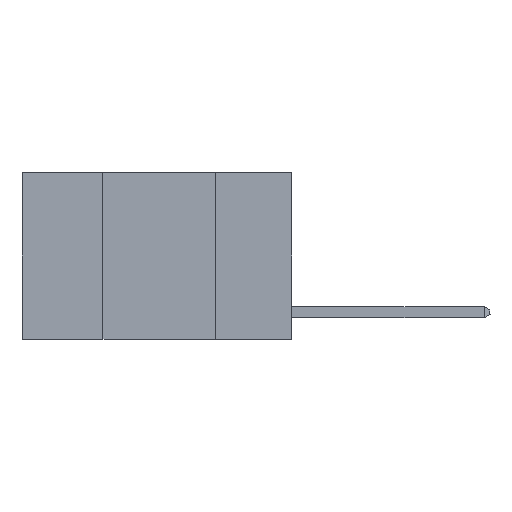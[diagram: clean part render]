
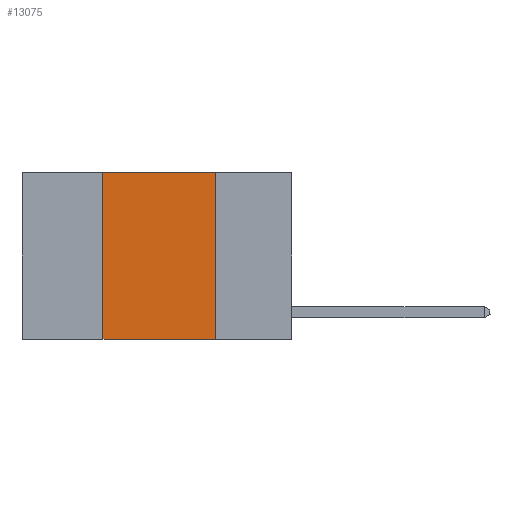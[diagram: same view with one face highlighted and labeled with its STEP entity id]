
A CAD part, left-side view. The second image highlights one B-rep face of the part: STEP entity #13075.
In plain terms, the highlighted planar face has unit normal (-1, 0, 0).
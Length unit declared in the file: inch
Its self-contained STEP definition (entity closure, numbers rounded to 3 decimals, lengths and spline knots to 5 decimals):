
#274 = VECTOR ( 'NONE', #16319, 39.37008 ) ;
#1256 = LINE ( 'NONE', #19214, #22501 ) ;
#1364 = CARTESIAN_POINT ( 'NONE',  ( 0., 0.17, 0. ) ) ;
#1908 = LINE ( 'NONE', #15973, #274 ) ;
#2144 = DIRECTION ( 'NONE',  ( 0., -1., 0. ) ) ;
#2211 = CARTESIAN_POINT ( 'NONE',  ( 0., 0.6, 0. ) ) ;
#2623 = CARTESIAN_POINT ( 'NONE',  ( 0., 0.42, 0. ) ) ;
#2859 = ORIENTED_EDGE ( 'NONE', *, *, #5533, .F. ) ;
#3332 = PLANE ( 'NONE',  #6863 ) ;
#3520 = ORIENTED_EDGE ( 'NONE', *, *, #22010, .F. ) ;
#4323 = VERTEX_POINT ( 'NONE', #11855 ) ;
#4763 = VERTEX_POINT ( 'NONE', #1364 ) ;
#4826 = CARTESIAN_POINT ( 'NONE',  ( 0., 0.6, 0. ) ) ;
#5484 = VECTOR ( 'NONE', #10722, 39.37008 ) ;
#5533 = EDGE_CURVE ( 'NONE', #20583, #4763, #5913, .T. ) ;
#5913 = LINE ( 'NONE', #2211, #5484 ) ;
#6428 = EDGE_CURVE ( 'NONE', #4323, #20583, #1256, .T. ) ;
#6863 = AXIS2_PLACEMENT_3D ( 'NONE', #4826, #11862, #8511 ) ;
#8511 = DIRECTION ( 'NONE',  ( 0., 0., -1. ) ) ;
#9166 = ORIENTED_EDGE ( 'NONE', *, *, #12781, .T. ) ;
#9820 = VECTOR ( 'NONE', #2144, 39.37008 ) ;
#10216 = ORIENTED_EDGE ( 'NONE', *, *, #6428, .F. ) ;
#10437 = DIRECTION ( 'NONE',  ( 0., 0., 1. ) ) ;
#10722 = DIRECTION ( 'NONE',  ( 0., -1., 0. ) ) ;
#11855 = CARTESIAN_POINT ( 'NONE',  ( 0., 0.42, -0.37 ) ) ;
#11862 = DIRECTION ( 'NONE',  ( 1., 0., 0. ) ) ;
#12766 = CARTESIAN_POINT ( 'NONE',  ( 0., 0.6, -0.37 ) ) ;
#12781 = EDGE_CURVE ( 'NONE', #4323, #16736, #14486, .T. ) ;
#13075 = ADVANCED_FACE ( 'NONE', ( #20639 ), #3332, .F. ) ;
#13975 = CARTESIAN_POINT ( 'NONE',  ( 0., 0.17, -0.37 ) ) ;
#14486 = LINE ( 'NONE', #12766, #9820 ) ;
#15973 = CARTESIAN_POINT ( 'NONE',  ( 0., 0.17, 0. ) ) ;
#16319 = DIRECTION ( 'NONE',  ( 0., 0., -1. ) ) ;
#16736 = VERTEX_POINT ( 'NONE', #13975 ) ;
#18454 = EDGE_LOOP ( 'NONE', ( #3520, #2859, #10216, #9166 ) ) ;
#19214 = CARTESIAN_POINT ( 'NONE',  ( 0., 0.42, 0. ) ) ;
#20583 = VERTEX_POINT ( 'NONE', #2623 ) ;
#20639 = FACE_OUTER_BOUND ( 'NONE', #18454, .T. ) ;
#22010 = EDGE_CURVE ( 'NONE', #4763, #16736, #1908, .T. ) ;
#22501 = VECTOR ( 'NONE', #10437, 39.37008 ) ;
